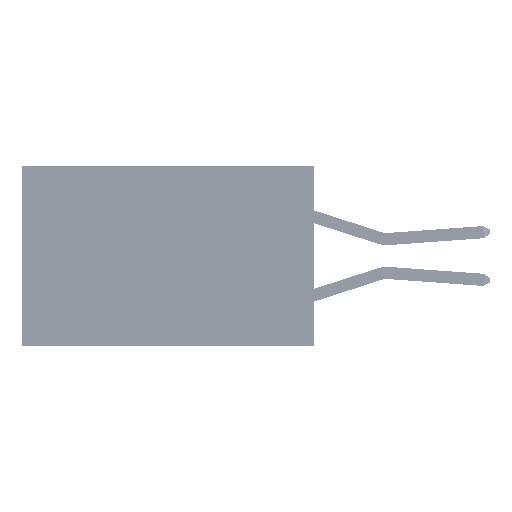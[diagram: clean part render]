
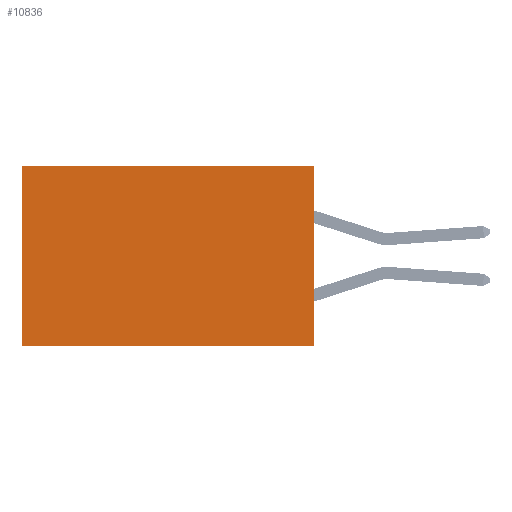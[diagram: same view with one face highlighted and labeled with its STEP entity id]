
A CAD part, left-side view. The second image highlights one B-rep face of the part: STEP entity #10836.
In plain terms, the highlighted planar face has unit normal (-1, 0, 0).
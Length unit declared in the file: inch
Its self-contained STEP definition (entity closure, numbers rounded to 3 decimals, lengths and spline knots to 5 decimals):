
#538 = CARTESIAN_POINT ( 'NONE',  ( 0.2875, 0., 0. ) ) ;
#1039 = VECTOR ( 'NONE', #27757, 39.37008 ) ;
#1574 = ORIENTED_EDGE ( 'NONE', *, *, #12435, .T. ) ;
#1736 = VERTEX_POINT ( 'NONE', #18285 ) ;
#1903 = EDGE_CURVE ( 'NONE', #25806, #1736, #33545, .T. ) ;
#2147 = LINE ( 'NONE', #24304, #1039 ) ;
#3854 = DIRECTION ( 'NONE',  ( 1., 0., 0. ) ) ;
#5756 = FACE_OUTER_BOUND ( 'NONE', #7133, .T. ) ;
#7133 = EDGE_LOOP ( 'NONE', ( #18707, #24357, #40716, #1574 ) ) ;
#8827 = VERTEX_POINT ( 'NONE', #41481 ) ;
#9558 = DIRECTION ( 'NONE',  ( 0., 0., -1. ) ) ;
#10836 = ADVANCED_FACE ( 'NONE', ( #5756 ), #32846, .F. ) ;
#11135 = VECTOR ( 'NONE', #9558, 39.37008 ) ;
#12175 = AXIS2_PLACEMENT_3D ( 'NONE', #538, #3854, #29198 ) ;
#12435 = EDGE_CURVE ( 'NONE', #25806, #8827, #43157, .T. ) ;
#12972 = EDGE_CURVE ( 'NONE', #8827, #19341, #22376, .T. ) ;
#15764 = CARTESIAN_POINT ( 'NONE',  ( 0.2875, 0.6, -0.37 ) ) ;
#17004 = DIRECTION ( 'NONE',  ( 0., 1., 0. ) ) ;
#18285 = CARTESIAN_POINT ( 'NONE',  ( 0.2875, 0., -0.37 ) ) ;
#18707 = ORIENTED_EDGE ( 'NONE', *, *, #12972, .T. ) ;
#19341 = VERTEX_POINT ( 'NONE', #15764 ) ;
#21852 = VECTOR ( 'NONE', #17004, 39.37008 ) ;
#22376 = LINE ( 'NONE', #27967, #39146 ) ;
#24304 = CARTESIAN_POINT ( 'NONE',  ( 0.2875, 0., -0.37 ) ) ;
#24357 = ORIENTED_EDGE ( 'NONE', *, *, #43854, .F. ) ;
#25806 = VERTEX_POINT ( 'NONE', #42001 ) ;
#27757 = DIRECTION ( 'NONE',  ( 0., 1., 0. ) ) ;
#27967 = CARTESIAN_POINT ( 'NONE',  ( 0.2875, 0.6, 0. ) ) ;
#29198 = DIRECTION ( 'NONE',  ( 0., 0., -1. ) ) ;
#32846 = PLANE ( 'NONE',  #12175 ) ;
#33545 = LINE ( 'NONE', #44210, #11135 ) ;
#38462 = CARTESIAN_POINT ( 'NONE',  ( 0.2875, 0., 0. ) ) ;
#39146 = VECTOR ( 'NONE', #43512, 39.37008 ) ;
#40716 = ORIENTED_EDGE ( 'NONE', *, *, #1903, .F. ) ;
#41481 = CARTESIAN_POINT ( 'NONE',  ( 0.2875, 0.6, 0. ) ) ;
#42001 = CARTESIAN_POINT ( 'NONE',  ( 0.2875, 0., 0. ) ) ;
#43157 = LINE ( 'NONE', #38462, #21852 ) ;
#43512 = DIRECTION ( 'NONE',  ( 0., 0., -1. ) ) ;
#43854 = EDGE_CURVE ( 'NONE', #1736, #19341, #2147, .T. ) ;
#44210 = CARTESIAN_POINT ( 'NONE',  ( 0.2875, 0., 0. ) ) ;
